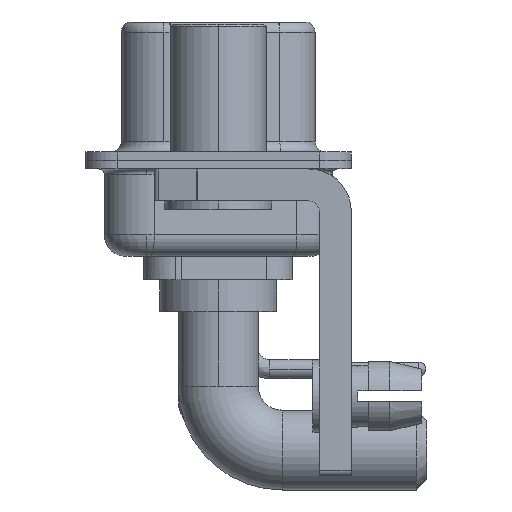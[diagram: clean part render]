
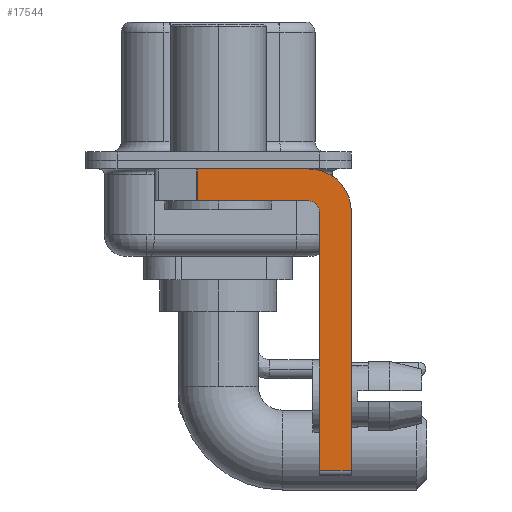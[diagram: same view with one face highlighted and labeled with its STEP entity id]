
A CAD part, left-side view. The second image highlights one B-rep face of the part: STEP entity #17544.
In plain terms, the highlighted planar face has unit normal (-1, 0, 0).
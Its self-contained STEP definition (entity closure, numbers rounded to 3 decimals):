
#4 = CARTESIAN_POINT ( 'NONE',  ( -2.9, -6.25, -2.4 ) ) ;
#51 = LINE ( 'NONE', #24410, #26043 ) ;
#253 = DIRECTION ( 'NONE',  ( 0., 0., 1. ) ) ;
#910 = DIRECTION ( 'NONE',  ( 0., -1., 0. ) ) ;
#1451 = VECTOR ( 'NONE', #30917, 1000. ) ;
#1539 = CARTESIAN_POINT ( 'NONE',  ( -2.9, -4.75, -2.4 ) ) ;
#1920 = CARTESIAN_POINT ( 'NONE',  ( -2.9, -6.25, -2.4 ) ) ;
#2396 = CARTESIAN_POINT ( 'NONE',  ( -2.9, 0.978, -0.4 ) ) ;
#3295 = EDGE_CURVE ( 'NONE', #19893, #20893, #27802, .T. ) ;
#3379 = VERTEX_POINT ( 'NONE', #1539 ) ;
#3840 = DIRECTION ( 'NONE',  ( 0., 0., -1. ) ) ;
#4081 = VERTEX_POINT ( 'NONE', #2396 ) ;
#4089 = EDGE_CURVE ( 'NONE', #16735, #5457, #22024, .T. ) ;
#4132 = FACE_OUTER_BOUND ( 'NONE', #25690, .T. ) ;
#4203 = CARTESIAN_POINT ( 'NONE',  ( -2.9, 0.978, -1.9 ) ) ;
#4947 = CARTESIAN_POINT ( 'NONE',  ( -2.9, 0.978, -1.9 ) ) ;
#5457 = VERTEX_POINT ( 'NONE', #4 ) ;
#6575 = LINE ( 'NONE', #30418, #13646 ) ;
#8114 = CARTESIAN_POINT ( 'NONE',  ( -2.9, -4.25, -14.55 ) ) ;
#8607 = CARTESIAN_POINT ( 'NONE',  ( -2.9, -4.25, -2.4 ) ) ;
#9261 = CARTESIAN_POINT ( 'NONE',  ( -2.9, -4.25, -2.4 ) ) ;
#9445 = CARTESIAN_POINT ( 'NONE',  ( -2.9, -6.25, -14.55 ) ) ;
#9979 = CARTESIAN_POINT ( 'NONE',  ( -2.9, -4.25, -2.4 ) ) ;
#10654 = VECTOR ( 'NONE', #24504, 1000. ) ;
#11227 = VECTOR ( 'NONE', #3840, 1000. ) ;
#12123 = AXIS2_PLACEMENT_3D ( 'NONE', #8607, #18304, #18782 ) ;
#12512 = CARTESIAN_POINT ( 'NONE',  ( -2.9, -4.25, -1.9 ) ) ;
#13251 = EDGE_CURVE ( 'NONE', #4081, #16735, #6575, .T. ) ;
#13491 = ORIENTED_EDGE ( 'NONE', *, *, #30781, .F. ) ;
#13646 = VECTOR ( 'NONE', #23093, 1000. ) ;
#13766 = VERTEX_POINT ( 'NONE', #12512 ) ;
#13905 = CARTESIAN_POINT ( 'NONE',  ( -2.9, -4.25, -1.9 ) ) ;
#14225 = ORIENTED_EDGE ( 'NONE', *, *, #15864, .F. ) ;
#14816 = ORIENTED_EDGE ( 'NONE', *, *, #4089, .F. ) ;
#15864 = EDGE_CURVE ( 'NONE', #5457, #20893, #20707, .T. ) ;
#16473 = ORIENTED_EDGE ( 'NONE', *, *, #20122, .T. ) ;
#16735 = VERTEX_POINT ( 'NONE', #17237 ) ;
#17237 = CARTESIAN_POINT ( 'NONE',  ( -2.9, -4.25, -0.4 ) ) ;
#17544 = ADVANCED_FACE ( 'NONE', ( #4132 ), #23531, .F. ) ;
#18011 = EDGE_CURVE ( 'NONE', #13766, #28470, #23595, .T. ) ;
#18304 = DIRECTION ( 'NONE',  ( 1., 0., 0. ) ) ;
#18689 = ORIENTED_EDGE ( 'NONE', *, *, #18011, .F. ) ;
#18782 = DIRECTION ( 'NONE',  ( 0., 0., -1. ) ) ;
#19573 = LINE ( 'NONE', #4947, #10654 ) ;
#19893 = VERTEX_POINT ( 'NONE', #23399 ) ;
#20122 = EDGE_CURVE ( 'NONE', #4081, #28470, #19573, .T. ) ;
#20707 = LINE ( 'NONE', #1920, #11227 ) ;
#20893 = VERTEX_POINT ( 'NONE', #9445 ) ;
#22024 = CIRCLE ( 'NONE', #25571, 2. ) ;
#23093 = DIRECTION ( 'NONE',  ( 0., -1., 0. ) ) ;
#23399 = CARTESIAN_POINT ( 'NONE',  ( -2.9, -4.75, -14.55 ) ) ;
#23531 = PLANE ( 'NONE',  #12123 ) ;
#23595 = LINE ( 'NONE', #13905, #1451 ) ;
#23784 = ORIENTED_EDGE ( 'NONE', *, *, #13251, .F. ) ;
#23971 = CIRCLE ( 'NONE', #25002, 0.5 ) ;
#24410 = CARTESIAN_POINT ( 'NONE',  ( -2.9, -4.75, -14.8 ) ) ;
#24504 = DIRECTION ( 'NONE',  ( 0., 0., -1. ) ) ;
#25002 = AXIS2_PLACEMENT_3D ( 'NONE', #9979, #29223, #253 ) ;
#25571 = AXIS2_PLACEMENT_3D ( 'NONE', #9261, #29131, #28811 ) ;
#25690 = EDGE_LOOP ( 'NONE', ( #23784, #16473, #18689, #28414, #13491, #31110, #14225, #14816 ) ) ;
#26043 = VECTOR ( 'NONE', #29645, 1000. ) ;
#26607 = VECTOR ( 'NONE', #910, 1000. ) ;
#27802 = LINE ( 'NONE', #8114, #26607 ) ;
#28414 = ORIENTED_EDGE ( 'NONE', *, *, #30302, .F. ) ;
#28470 = VERTEX_POINT ( 'NONE', #4203 ) ;
#28811 = DIRECTION ( 'NONE',  ( 0., 0., -1. ) ) ;
#29131 = DIRECTION ( 'NONE',  ( 1., 0., 0. ) ) ;
#29223 = DIRECTION ( 'NONE',  ( -1., 0., 0. ) ) ;
#29645 = DIRECTION ( 'NONE',  ( 0., 0., 1. ) ) ;
#30302 = EDGE_CURVE ( 'NONE', #3379, #13766, #23971, .T. ) ;
#30418 = CARTESIAN_POINT ( 'NONE',  ( -2.9, 3., -0.4 ) ) ;
#30781 = EDGE_CURVE ( 'NONE', #19893, #3379, #51, .T. ) ;
#30917 = DIRECTION ( 'NONE',  ( 0., 1., 0. ) ) ;
#31110 = ORIENTED_EDGE ( 'NONE', *, *, #3295, .T. ) ;
